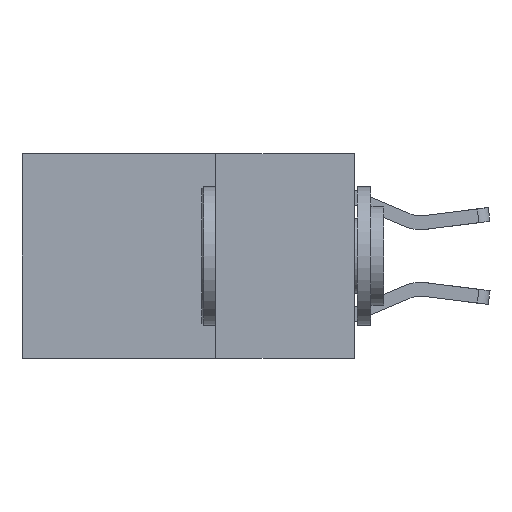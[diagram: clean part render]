
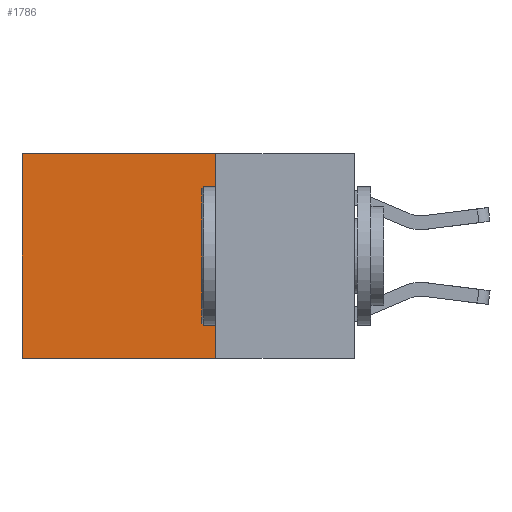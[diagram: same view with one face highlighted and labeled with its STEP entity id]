
A CAD part, left-side view. The second image highlights one B-rep face of the part: STEP entity #1786.
In plain terms, the highlighted planar face has unit normal (-1, 0, 0).
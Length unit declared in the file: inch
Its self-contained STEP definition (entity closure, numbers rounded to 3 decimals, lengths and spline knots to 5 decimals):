
#5 = DIRECTION ( 'NONE',  ( 0., 0., -1. ) ) ;
#437 = VECTOR ( 'NONE', #3871, 39.37008 ) ;
#888 = ORIENTED_EDGE ( 'NONE', *, *, #11763, .T. ) ;
#1289 = DIRECTION ( 'NONE',  ( 0., 0., -1. ) ) ;
#1291 = LINE ( 'NONE', #7141, #9293 ) ;
#1312 = LINE ( 'NONE', #4892, #9020 ) ;
#1786 = ADVANCED_FACE ( 'NONE', ( #2839 ), #7822, .F. ) ;
#1853 = ORIENTED_EDGE ( 'NONE', *, *, #4513, .T. ) ;
#2839 = FACE_OUTER_BOUND ( 'NONE', #7563, .T. ) ;
#2885 = CARTESIAN_POINT ( 'NONE',  ( 0.2625, 0.25, 0. ) ) ;
#3167 = VECTOR ( 'NONE', #5514, 39.37008 ) ;
#3216 = VERTEX_POINT ( 'NONE', #6040 ) ;
#3451 = CARTESIAN_POINT ( 'NONE',  ( 0.2625, 0.25, -0.37 ) ) ;
#3871 = DIRECTION ( 'NONE',  ( 0., 1., 0. ) ) ;
#4513 = EDGE_CURVE ( 'NONE', #10339, #3216, #6335, .T. ) ;
#4892 = CARTESIAN_POINT ( 'NONE',  ( 0.2625, 0.25, -0.37 ) ) ;
#5048 = CARTESIAN_POINT ( 'NONE',  ( 0.2625, 0.25, 0. ) ) ;
#5514 = DIRECTION ( 'NONE',  ( 0., 0., -1. ) ) ;
#5851 = VERTEX_POINT ( 'NONE', #7763 ) ;
#5988 = DIRECTION ( 'NONE',  ( 1., 0., 0. ) ) ;
#6040 = CARTESIAN_POINT ( 'NONE',  ( 0.2625, 0.6, 0. ) ) ;
#6059 = ORIENTED_EDGE ( 'NONE', *, *, #9366, .F. ) ;
#6335 = LINE ( 'NONE', #2885, #437 ) ;
#7141 = CARTESIAN_POINT ( 'NONE',  ( 0.2625, 0.6, 0. ) ) ;
#7563 = EDGE_LOOP ( 'NONE', ( #888, #10726, #6059, #1853 ) ) ;
#7763 = CARTESIAN_POINT ( 'NONE',  ( 0.2625, 0.6, -0.37 ) ) ;
#7822 = PLANE ( 'NONE',  #8115 ) ;
#8115 = AXIS2_PLACEMENT_3D ( 'NONE', #11493, #5988, #5 ) ;
#9020 = VECTOR ( 'NONE', #12225, 39.37008 ) ;
#9293 = VECTOR ( 'NONE', #1289, 39.37008 ) ;
#9366 = EDGE_CURVE ( 'NONE', #10339, #11174, #10395, .T. ) ;
#10339 = VERTEX_POINT ( 'NONE', #5048 ) ;
#10395 = LINE ( 'NONE', #11045, #3167 ) ;
#10726 = ORIENTED_EDGE ( 'NONE', *, *, #11488, .F. ) ;
#11045 = CARTESIAN_POINT ( 'NONE',  ( 0.2625, 0.25, 0. ) ) ;
#11174 = VERTEX_POINT ( 'NONE', #3451 ) ;
#11488 = EDGE_CURVE ( 'NONE', #11174, #5851, #1312, .T. ) ;
#11493 = CARTESIAN_POINT ( 'NONE',  ( 0.2625, 0.25, 0. ) ) ;
#11763 = EDGE_CURVE ( 'NONE', #3216, #5851, #1291, .T. ) ;
#12225 = DIRECTION ( 'NONE',  ( 0., 1., 0. ) ) ;
